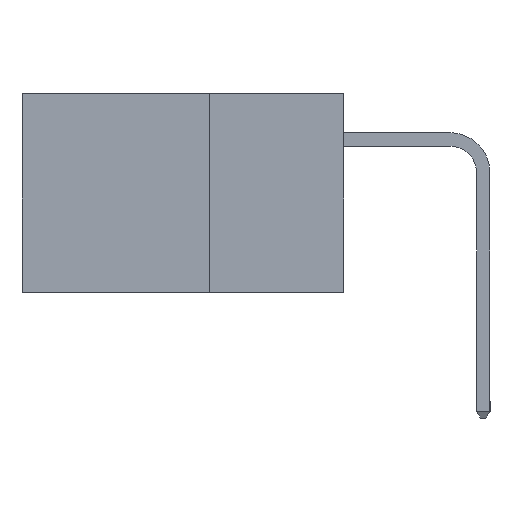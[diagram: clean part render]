
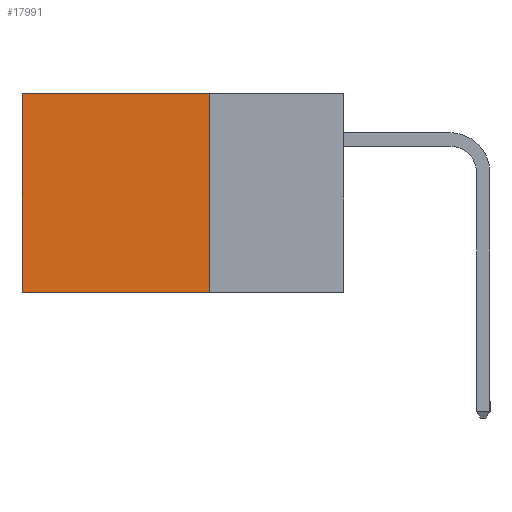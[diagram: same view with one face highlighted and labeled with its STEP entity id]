
A CAD part, left-side view. The second image highlights one B-rep face of the part: STEP entity #17991.
In plain terms, the highlighted planar face has unit normal (-1, 0, 0).
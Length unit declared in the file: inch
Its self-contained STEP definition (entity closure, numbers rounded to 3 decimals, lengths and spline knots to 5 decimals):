
#139 = VERTEX_POINT ( 'NONE', #12732 ) ;
#143 = FACE_OUTER_BOUND ( 'NONE', #17837, .T. ) ;
#858 = ORIENTED_EDGE ( 'NONE', *, *, #13335, .F. ) ;
#1376 = ORIENTED_EDGE ( 'NONE', *, *, #8233, .T. ) ;
#1399 = LINE ( 'NONE', #9105, #4437 ) ;
#1436 = DIRECTION ( 'NONE',  ( 0., 0., -1. ) ) ;
#1480 = LINE ( 'NONE', #9082, #16904 ) ;
#1524 = CARTESIAN_POINT ( 'NONE',  ( 0.2615, 0.25, -0.37 ) ) ;
#1767 = DIRECTION ( 'NONE',  ( 0., 0., -1. ) ) ;
#2817 = CARTESIAN_POINT ( 'NONE',  ( 0.2615, 0.25, -0.37 ) ) ;
#3983 = CARTESIAN_POINT ( 'NONE',  ( 0.2615, 0.6, 0. ) ) ;
#4437 = VECTOR ( 'NONE', #1767, 39.37008 ) ;
#5776 = DIRECTION ( 'NONE',  ( 0., 0., -1. ) ) ;
#6119 = CARTESIAN_POINT ( 'NONE',  ( 0.2615, 0.25, 0. ) ) ;
#6231 = ORIENTED_EDGE ( 'NONE', *, *, #8898, .F. ) ;
#8050 = CARTESIAN_POINT ( 'NONE',  ( 0.2615, 0.25, -0.37 ) ) ;
#8233 = EDGE_CURVE ( 'NONE', #16522, #12866, #1480, .T. ) ;
#8898 = EDGE_CURVE ( 'NONE', #16522, #139, #17111, .T. ) ;
#8986 = DIRECTION ( 'NONE',  ( 0., 1., 0. ) ) ;
#9082 = CARTESIAN_POINT ( 'NONE',  ( 0.2615, 0.25, 0. ) ) ;
#9105 = CARTESIAN_POINT ( 'NONE',  ( 0.2615, 0.6, -0.37 ) ) ;
#10041 = EDGE_CURVE ( 'NONE', #12866, #16534, #1399, .T. ) ;
#12732 = CARTESIAN_POINT ( 'NONE',  ( 0.2615, 0.25, -0.37 ) ) ;
#12866 = VERTEX_POINT ( 'NONE', #3983 ) ;
#13114 = ORIENTED_EDGE ( 'NONE', *, *, #10041, .T. ) ;
#13256 = PLANE ( 'NONE',  #13920 ) ;
#13335 = EDGE_CURVE ( 'NONE', #139, #16534, #13768, .T. ) ;
#13652 = CARTESIAN_POINT ( 'NONE',  ( 0.2615, 0.6, -0.37 ) ) ;
#13768 = LINE ( 'NONE', #8050, #17705 ) ;
#13920 = AXIS2_PLACEMENT_3D ( 'NONE', #2817, #14730, #5776 ) ;
#14730 = DIRECTION ( 'NONE',  ( 1., 0., 0. ) ) ;
#16522 = VERTEX_POINT ( 'NONE', #6119 ) ;
#16534 = VERTEX_POINT ( 'NONE', #13652 ) ;
#16642 = VECTOR ( 'NONE', #1436, 39.37008 ) ;
#16904 = VECTOR ( 'NONE', #8986, 39.37008 ) ;
#17111 = LINE ( 'NONE', #1524, #16642 ) ;
#17705 = VECTOR ( 'NONE', #18476, 39.37008 ) ;
#17837 = EDGE_LOOP ( 'NONE', ( #13114, #858, #6231, #1376 ) ) ;
#17991 = ADVANCED_FACE ( 'NONE', ( #143 ), #13256, .F. ) ;
#18476 = DIRECTION ( 'NONE',  ( 0., 1., 0. ) ) ;
